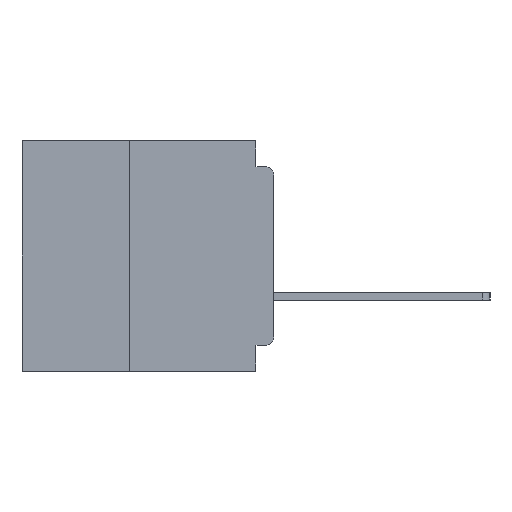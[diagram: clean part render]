
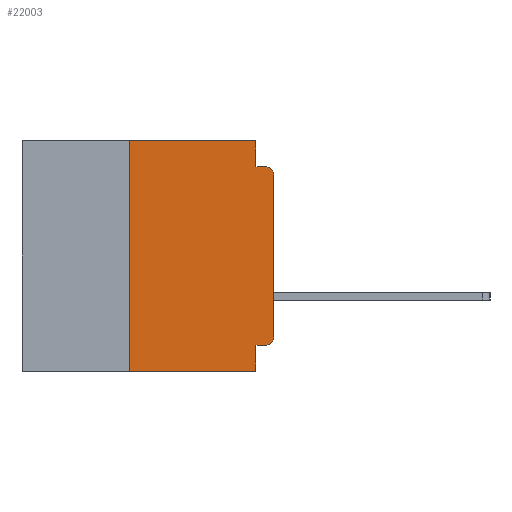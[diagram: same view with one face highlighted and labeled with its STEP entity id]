
A CAD part, left-side view. The second image highlights one B-rep face of the part: STEP entity #22003.
In plain terms, the highlighted planar face has unit normal (-1, 0, 0).
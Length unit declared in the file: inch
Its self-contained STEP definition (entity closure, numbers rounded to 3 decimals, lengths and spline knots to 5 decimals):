
#1281 = FACE_OUTER_BOUND ( 'NONE', #27758, .T. ) ;
#1356 = VERTEX_POINT ( 'NONE', #29258 ) ;
#1403 = VECTOR ( 'NONE', #36529, 39.37008 ) ;
#1998 = LINE ( 'NONE', #37511, #21046 ) ;
#2957 = CARTESIAN_POINT ( 'NONE',  ( 0., 0., -0.34 ) ) ;
#3095 = DIRECTION ( 'NONE',  ( 0., 0., -1. ) ) ;
#3937 = ORIENTED_EDGE ( 'NONE', *, *, #10579, .T. ) ;
#4475 = CARTESIAN_POINT ( 'NONE',  ( 0., 0.25, -0.4 ) ) ;
#5884 = ORIENTED_EDGE ( 'NONE', *, *, #26133, .T. ) ;
#6133 = CARTESIAN_POINT ( 'NONE',  ( 0., 0.031, -0.355 ) ) ;
#6830 = ORIENTED_EDGE ( 'NONE', *, *, #45348, .T. ) ;
#7688 = CARTESIAN_POINT ( 'NONE',  ( 0., 0.031, 0. ) ) ;
#8418 = AXIS2_PLACEMENT_3D ( 'NONE', #32526, #11034, #36134 ) ;
#9791 = VERTEX_POINT ( 'NONE', #2957 ) ;
#10036 = CARTESIAN_POINT ( 'NONE',  ( 0., 0.031, -0.045 ) ) ;
#10579 = EDGE_CURVE ( 'NONE', #9791, #44518, #31763, .T. ) ;
#10623 = ORIENTED_EDGE ( 'NONE', *, *, #40796, .F. ) ;
#10801 = CARTESIAN_POINT ( 'NONE',  ( 0., 0., -0.06 ) ) ;
#10952 = LINE ( 'NONE', #11436, #1403 ) ;
#11034 = DIRECTION ( 'NONE',  ( 1., 0., 0. ) ) ;
#11436 = CARTESIAN_POINT ( 'NONE',  ( 0., 0.031, -0.4 ) ) ;
#11483 = EDGE_CURVE ( 'NONE', #33815, #43144, #12582, .T. ) ;
#11963 = EDGE_CURVE ( 'NONE', #25073, #14642, #10952, .T. ) ;
#12346 = CARTESIAN_POINT ( 'NONE',  ( 0., 0.015, -0.34 ) ) ;
#12378 = ORIENTED_EDGE ( 'NONE', *, *, #11963, .F. ) ;
#12582 = LINE ( 'NONE', #33741, #30535 ) ;
#12673 = VECTOR ( 'NONE', #14938, 39.37008 ) ;
#13721 = CIRCLE ( 'NONE', #38050, 0.015 ) ;
#13746 = VERTEX_POINT ( 'NONE', #7688 ) ;
#14642 = VERTEX_POINT ( 'NONE', #26545 ) ;
#14938 = DIRECTION ( 'NONE',  ( 0., 0., 1. ) ) ;
#15052 = CARTESIAN_POINT ( 'NONE',  ( 0., 0.031, 0. ) ) ;
#15913 = DIRECTION ( 'NONE',  ( 0., 0., -1. ) ) ;
#15977 = DIRECTION ( 'NONE',  ( 0., 0., 1. ) ) ;
#16709 = EDGE_CURVE ( 'NONE', #24107, #14642, #17945, .T. ) ;
#17945 = LINE ( 'NONE', #24468, #19058 ) ;
#18517 = CARTESIAN_POINT ( 'NONE',  ( 0., 0., 0. ) ) ;
#18541 = CARTESIAN_POINT ( 'NONE',  ( 0., 0., -0.355 ) ) ;
#19058 = VECTOR ( 'NONE', #45948, 39.37008 ) ;
#20459 = ORIENTED_EDGE ( 'NONE', *, *, #33613, .F. ) ;
#20492 = AXIS2_PLACEMENT_3D ( 'NONE', #12346, #37451, #15913 ) ;
#21046 = VECTOR ( 'NONE', #15977, 39.37008 ) ;
#22003 = ADVANCED_FACE ( 'NONE', ( #1281 ), #25258, .F. ) ;
#22185 = LINE ( 'NONE', #18541, #24411 ) ;
#24107 = VERTEX_POINT ( 'NONE', #4475 ) ;
#24411 = VECTOR ( 'NONE', #33049, 39.37008 ) ;
#24468 = CARTESIAN_POINT ( 'NONE',  ( 0., 0.437, -0.4 ) ) ;
#24534 = DIRECTION ( 'NONE',  ( -1., 0., 0. ) ) ;
#24852 = VECTOR ( 'NONE', #36592, 39.37008 ) ;
#25073 = VERTEX_POINT ( 'NONE', #6133 ) ;
#25258 = PLANE ( 'NONE',  #8418 ) ;
#25659 = ORIENTED_EDGE ( 'NONE', *, *, #11483, .F. ) ;
#25863 = VECTOR ( 'NONE', #43453, 39.37008 ) ;
#26133 = EDGE_CURVE ( 'NONE', #27833, #9791, #44596, .T. ) ;
#26545 = CARTESIAN_POINT ( 'NONE',  ( 0., 0.031, -0.4 ) ) ;
#27758 = EDGE_LOOP ( 'NONE', ( #3937, #6830, #25659, #10623, #42935, #20459, #45409, #12378, #30723, #5884 ) ) ;
#27833 = VERTEX_POINT ( 'NONE', #40739 ) ;
#29258 = CARTESIAN_POINT ( 'NONE',  ( 0., 0.25, 0. ) ) ;
#30065 = EDGE_CURVE ( 'NONE', #27833, #25073, #22185, .T. ) ;
#30535 = VECTOR ( 'NONE', #37342, 39.37008 ) ;
#30723 = ORIENTED_EDGE ( 'NONE', *, *, #30065, .F. ) ;
#31763 = LINE ( 'NONE', #18517, #12673 ) ;
#32526 = CARTESIAN_POINT ( 'NONE',  ( 0., 0.437, 0. ) ) ;
#33049 = DIRECTION ( 'NONE',  ( 0., 1., 0. ) ) ;
#33613 = EDGE_CURVE ( 'NONE', #24107, #1356, #1998, .T. ) ;
#33741 = CARTESIAN_POINT ( 'NONE',  ( 0., 0., -0.045 ) ) ;
#33815 = VERTEX_POINT ( 'NONE', #10036 ) ;
#34448 = LINE ( 'NONE', #15052, #24852 ) ;
#35240 = CARTESIAN_POINT ( 'NONE',  ( 0., 0.015, -0.045 ) ) ;
#36134 = DIRECTION ( 'NONE',  ( 0., 0., -1. ) ) ;
#36454 = CARTESIAN_POINT ( 'NONE',  ( 0., 0.437, 0. ) ) ;
#36511 = EDGE_CURVE ( 'NONE', #1356, #13746, #36595, .T. ) ;
#36529 = DIRECTION ( 'NONE',  ( 0., 0., -1. ) ) ;
#36592 = DIRECTION ( 'NONE',  ( 0., 0., -1. ) ) ;
#36595 = LINE ( 'NONE', #36454, #25863 ) ;
#37342 = DIRECTION ( 'NONE',  ( 0., -1., 0. ) ) ;
#37451 = DIRECTION ( 'NONE',  ( -1., 0., 0. ) ) ;
#37511 = CARTESIAN_POINT ( 'NONE',  ( 0., 0.25, -0.4 ) ) ;
#38050 = AXIS2_PLACEMENT_3D ( 'NONE', #46007, #24534, #3095 ) ;
#40739 = CARTESIAN_POINT ( 'NONE',  ( 0., 0.015, -0.355 ) ) ;
#40796 = EDGE_CURVE ( 'NONE', #13746, #33815, #34448, .T. ) ;
#42935 = ORIENTED_EDGE ( 'NONE', *, *, #36511, .F. ) ;
#43144 = VERTEX_POINT ( 'NONE', #35240 ) ;
#43453 = DIRECTION ( 'NONE',  ( 0., -1., 0. ) ) ;
#44518 = VERTEX_POINT ( 'NONE', #10801 ) ;
#44596 = CIRCLE ( 'NONE', #20492, 0.015 ) ;
#45348 = EDGE_CURVE ( 'NONE', #44518, #43144, #13721, .T. ) ;
#45409 = ORIENTED_EDGE ( 'NONE', *, *, #16709, .T. ) ;
#45948 = DIRECTION ( 'NONE',  ( 0., -1., 0. ) ) ;
#46007 = CARTESIAN_POINT ( 'NONE',  ( 0., 0.015, -0.06 ) ) ;
